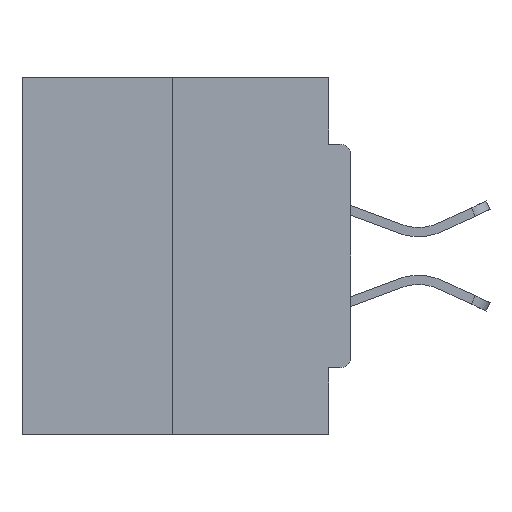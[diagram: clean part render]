
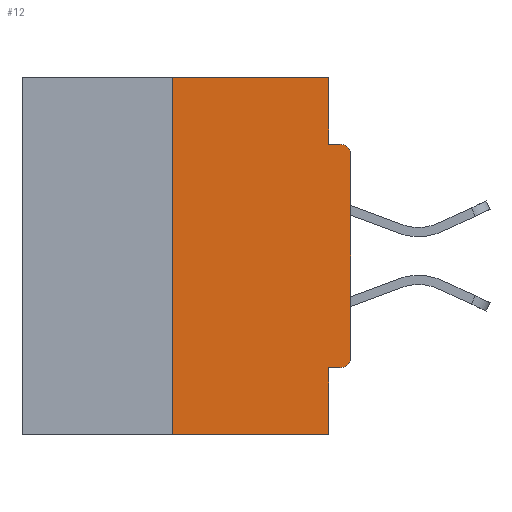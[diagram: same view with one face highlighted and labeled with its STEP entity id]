
A CAD part, left-side view. The second image highlights one B-rep face of the part: STEP entity #12.
In plain terms, the highlighted planar face has unit normal (-1, 0, 0).
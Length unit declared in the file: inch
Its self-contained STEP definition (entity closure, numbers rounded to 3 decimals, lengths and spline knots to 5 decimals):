
#12 = ADVANCED_FACE ( 'NONE', ( #30269 ), #18904, .F. ) ;
#523 = EDGE_CURVE ( 'NONE', #22866, #16379, #27816, .T. ) ;
#728 = LINE ( 'NONE', #26954, #32545 ) ;
#901 = CARTESIAN_POINT ( 'NONE',  ( 0., 0.031, -0.0935 ) ) ;
#1227 = ORIENTED_EDGE ( 'NONE', *, *, #7768, .F. ) ;
#1714 = CARTESIAN_POINT ( 'NONE',  ( 0., 0., -0.4065 ) ) ;
#1821 = ORIENTED_EDGE ( 'NONE', *, *, #24436, .F. ) ;
#2195 = EDGE_CURVE ( 'NONE', #28704, #2935, #23118, .T. ) ;
#2613 = CARTESIAN_POINT ( 'NONE',  ( 0., 0.031, -0.4065 ) ) ;
#2935 = VERTEX_POINT ( 'NONE', #26729 ) ;
#4211 = EDGE_CURVE ( 'NONE', #31020, #11159, #11793, .T. ) ;
#4270 = DIRECTION ( 'NONE',  ( 0., -1., 0. ) ) ;
#4783 = VECTOR ( 'NONE', #31444, 39.37008 ) ;
#5480 = AXIS2_PLACEMENT_3D ( 'NONE', #34135, #28930, #10332 ) ;
#5644 = ORIENTED_EDGE ( 'NONE', *, *, #16191, .F. ) ;
#5742 = DIRECTION ( 'NONE',  ( 0., 0., -1. ) ) ;
#5848 = CARTESIAN_POINT ( 'NONE',  ( 0., 0.031, -0.5 ) ) ;
#6681 = VECTOR ( 'NONE', #17038, 39.37008 ) ;
#6756 = ORIENTED_EDGE ( 'NONE', *, *, #23557, .F. ) ;
#7768 = EDGE_CURVE ( 'NONE', #25973, #27434, #18005, .T. ) ;
#7908 = VECTOR ( 'NONE', #26815, 39.37008 ) ;
#8691 = ORIENTED_EDGE ( 'NONE', *, *, #523, .F. ) ;
#9714 = CARTESIAN_POINT ( 'NONE',  ( 0., 0.015, -0.1085 ) ) ;
#9810 = CARTESIAN_POINT ( 'NONE',  ( 0., 0.25, 0. ) ) ;
#10106 = CARTESIAN_POINT ( 'NONE',  ( 0., 0.25, 0. ) ) ;
#10201 = CARTESIAN_POINT ( 'NONE',  ( 0., 0.46, 0. ) ) ;
#10332 = DIRECTION ( 'NONE',  ( 0., 0., -1. ) ) ;
#10497 = CARTESIAN_POINT ( 'NONE',  ( 0., 0., 0. ) ) ;
#10664 = EDGE_CURVE ( 'NONE', #32496, #16379, #33523, .T. ) ;
#11159 = VERTEX_POINT ( 'NONE', #5848 ) ;
#11793 = LINE ( 'NONE', #14442, #18798 ) ;
#12102 = CARTESIAN_POINT ( 'NONE',  ( 0., 0., -0.1085 ) ) ;
#12698 = DIRECTION ( 'NONE',  ( 0., 0., -1. ) ) ;
#12869 = DIRECTION ( 'NONE',  ( 0., 0., 1. ) ) ;
#13028 = DIRECTION ( 'NONE',  ( 0., 0., 1. ) ) ;
#13294 = CARTESIAN_POINT ( 'NONE',  ( 0., 0., -0.0935 ) ) ;
#14290 = EDGE_CURVE ( 'NONE', #2935, #32496, #29544, .T. ) ;
#14442 = CARTESIAN_POINT ( 'NONE',  ( 0., 0.46, -0.5 ) ) ;
#14892 = DIRECTION ( 'NONE',  ( -1., 0., 0. ) ) ;
#15009 = CARTESIAN_POINT ( 'NONE',  ( 0., 0.015, -0.0935 ) ) ;
#15623 = ORIENTED_EDGE ( 'NONE', *, *, #15976, .F. ) ;
#15845 = DIRECTION ( 'NONE',  ( 0., -1., 0. ) ) ;
#15976 = EDGE_CURVE ( 'NONE', #28704, #22652, #17001, .T. ) ;
#16191 = EDGE_CURVE ( 'NONE', #22652, #11159, #28158, .T. ) ;
#16237 = ORIENTED_EDGE ( 'NONE', *, *, #4211, .T. ) ;
#16295 = DIRECTION ( 'NONE',  ( 0., 0., -1. ) ) ;
#16379 = VERTEX_POINT ( 'NONE', #15009 ) ;
#16966 = CARTESIAN_POINT ( 'NONE',  ( 0., 0.031, 0. ) ) ;
#17001 = LINE ( 'NONE', #1714, #6681 ) ;
#17038 = DIRECTION ( 'NONE',  ( 0., 1., 0. ) ) ;
#17693 = LINE ( 'NONE', #10106, #28047 ) ;
#17906 = EDGE_LOOP ( 'NONE', ( #1227, #6756, #16237, #5644, #15623, #20536, #20979, #20814, #8691, #1821 ) ) ;
#18005 = LINE ( 'NONE', #10201, #4783 ) ;
#18798 = VECTOR ( 'NONE', #4270, 39.37008 ) ;
#18904 = PLANE ( 'NONE',  #33123 ) ;
#19017 = CARTESIAN_POINT ( 'NONE',  ( 0., 0.46, 0. ) ) ;
#20536 = ORIENTED_EDGE ( 'NONE', *, *, #2195, .T. ) ;
#20814 = ORIENTED_EDGE ( 'NONE', *, *, #10664, .T. ) ;
#20979 = ORIENTED_EDGE ( 'NONE', *, *, #14290, .T. ) ;
#22444 = VECTOR ( 'NONE', #15845, 39.37008 ) ;
#22652 = VERTEX_POINT ( 'NONE', #2613 ) ;
#22866 = VERTEX_POINT ( 'NONE', #901 ) ;
#23118 = CIRCLE ( 'NONE', #5480, 0.015 ) ;
#23557 = EDGE_CURVE ( 'NONE', #31020, #25973, #17693, .T. ) ;
#24238 = CARTESIAN_POINT ( 'NONE',  ( 0., 0.031, -0.5 ) ) ;
#24436 = EDGE_CURVE ( 'NONE', #27434, #22866, #728, .T. ) ;
#24483 = CARTESIAN_POINT ( 'NONE',  ( 0., 0.25, -0.5 ) ) ;
#25973 = VERTEX_POINT ( 'NONE', #9810 ) ;
#26693 = CARTESIAN_POINT ( 'NONE',  ( 0., 0.015, -0.4065 ) ) ;
#26729 = CARTESIAN_POINT ( 'NONE',  ( 0., 0., -0.3915 ) ) ;
#26815 = DIRECTION ( 'NONE',  ( 0., 0., -1. ) ) ;
#26954 = CARTESIAN_POINT ( 'NONE',  ( 0., 0.031, 0. ) ) ;
#27078 = VECTOR ( 'NONE', #13028, 39.37008 ) ;
#27434 = VERTEX_POINT ( 'NONE', #16966 ) ;
#27816 = LINE ( 'NONE', #13294, #22444 ) ;
#28047 = VECTOR ( 'NONE', #12869, 39.37008 ) ;
#28158 = LINE ( 'NONE', #24238, #7908 ) ;
#28704 = VERTEX_POINT ( 'NONE', #26693 ) ;
#28930 = DIRECTION ( 'NONE',  ( -1., 0., 0. ) ) ;
#29544 = LINE ( 'NONE', #10497, #27078 ) ;
#30269 = FACE_OUTER_BOUND ( 'NONE', #17906, .T. ) ;
#31020 = VERTEX_POINT ( 'NONE', #24483 ) ;
#31444 = DIRECTION ( 'NONE',  ( 0., -1., 0. ) ) ;
#31530 = AXIS2_PLACEMENT_3D ( 'NONE', #9714, #14892, #12698 ) ;
#32321 = DIRECTION ( 'NONE',  ( 1., 0., 0. ) ) ;
#32496 = VERTEX_POINT ( 'NONE', #12102 ) ;
#32545 = VECTOR ( 'NONE', #16295, 39.37008 ) ;
#33123 = AXIS2_PLACEMENT_3D ( 'NONE', #19017, #32321, #5742 ) ;
#33523 = CIRCLE ( 'NONE', #31530, 0.015 ) ;
#34135 = CARTESIAN_POINT ( 'NONE',  ( 0., 0.015, -0.3915 ) ) ;
